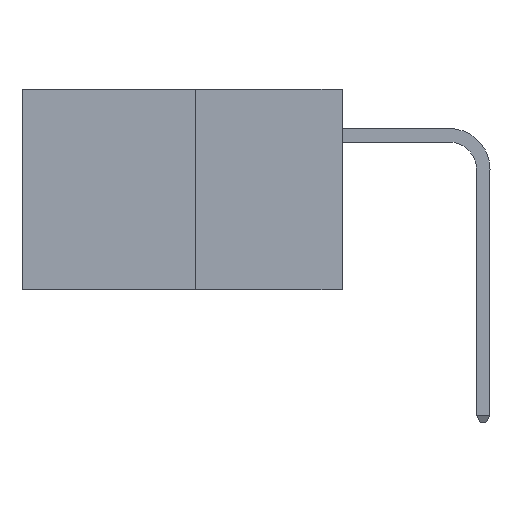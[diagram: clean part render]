
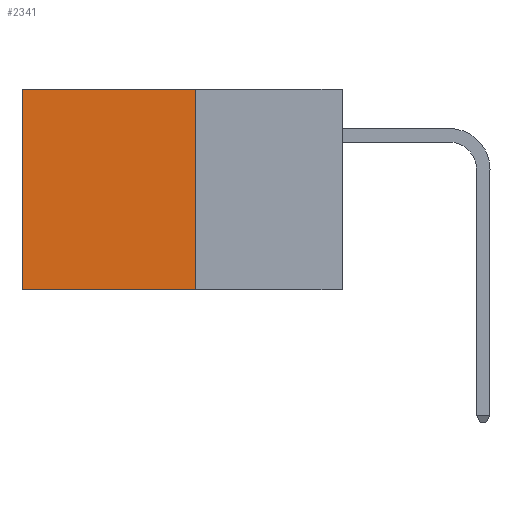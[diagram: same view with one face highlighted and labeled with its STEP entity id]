
A CAD part, left-side view. The second image highlights one B-rep face of the part: STEP entity #2341.
In plain terms, the highlighted planar face has unit normal (-1, 0, 0).
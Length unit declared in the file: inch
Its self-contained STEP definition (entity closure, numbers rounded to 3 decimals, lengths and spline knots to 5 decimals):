
#667 = EDGE_CURVE ( 'NONE', #9283, #12226, #4034, .T. ) ;
#782 = CARTESIAN_POINT ( 'NONE',  ( 0.277, 0.27, -0.37 ) ) ;
#2341 = ADVANCED_FACE ( 'NONE', ( #12576 ), #3841, .F. ) ;
#2682 = EDGE_CURVE ( 'NONE', #4708, #9283, #7208, .T. ) ;
#3140 = VECTOR ( 'NONE', #12223, 39.37008 ) ;
#3430 = LINE ( 'NONE', #12045, #8279 ) ;
#3554 = DIRECTION ( 'NONE',  ( 1., 0., 0. ) ) ;
#3633 = ORIENTED_EDGE ( 'NONE', *, *, #6909, .T. ) ;
#3764 = ORIENTED_EDGE ( 'NONE', *, *, #667, .F. ) ;
#3841 = PLANE ( 'NONE',  #4965 ) ;
#4034 = LINE ( 'NONE', #7117, #8804 ) ;
#4057 = EDGE_LOOP ( 'NONE', ( #3633, #3764, #4148, #4914 ) ) ;
#4108 = LINE ( 'NONE', #11892, #3140 ) ;
#4148 = ORIENTED_EDGE ( 'NONE', *, *, #2682, .F. ) ;
#4708 = VERTEX_POINT ( 'NONE', #10575 ) ;
#4914 = ORIENTED_EDGE ( 'NONE', *, *, #5161, .T. ) ;
#4965 = AXIS2_PLACEMENT_3D ( 'NONE', #7876, #3554, #12066 ) ;
#5161 = EDGE_CURVE ( 'NONE', #4708, #10980, #4108, .T. ) ;
#6490 = DIRECTION ( 'NONE',  ( 0., 1., 0. ) ) ;
#6909 = EDGE_CURVE ( 'NONE', #10980, #12226, #3430, .T. ) ;
#7117 = CARTESIAN_POINT ( 'NONE',  ( 0.277, 0.27, -0.37 ) ) ;
#7208 = LINE ( 'NONE', #11867, #9386 ) ;
#7876 = CARTESIAN_POINT ( 'NONE',  ( 0.277, 0.27, -0.37 ) ) ;
#8279 = VECTOR ( 'NONE', #8467, 39.37008 ) ;
#8467 = DIRECTION ( 'NONE',  ( 0., 0., -1. ) ) ;
#8804 = VECTOR ( 'NONE', #6490, 39.37008 ) ;
#9283 = VERTEX_POINT ( 'NONE', #782 ) ;
#9386 = VECTOR ( 'NONE', #9951, 39.37008 ) ;
#9951 = DIRECTION ( 'NONE',  ( 0., 0., -1. ) ) ;
#10575 = CARTESIAN_POINT ( 'NONE',  ( 0.277, 0.27, 0. ) ) ;
#10980 = VERTEX_POINT ( 'NONE', #11591 ) ;
#11591 = CARTESIAN_POINT ( 'NONE',  ( 0.277, 0.59, 0. ) ) ;
#11867 = CARTESIAN_POINT ( 'NONE',  ( 0.277, 0.27, -0.37 ) ) ;
#11892 = CARTESIAN_POINT ( 'NONE',  ( 0.277, 0.27, 0. ) ) ;
#12045 = CARTESIAN_POINT ( 'NONE',  ( 0.277, 0.59, -0.37 ) ) ;
#12066 = DIRECTION ( 'NONE',  ( 0., 0., -1. ) ) ;
#12223 = DIRECTION ( 'NONE',  ( 0., 1., 0. ) ) ;
#12226 = VERTEX_POINT ( 'NONE', #12472 ) ;
#12472 = CARTESIAN_POINT ( 'NONE',  ( 0.277, 0.59, -0.37 ) ) ;
#12576 = FACE_OUTER_BOUND ( 'NONE', #4057, .T. ) ;
